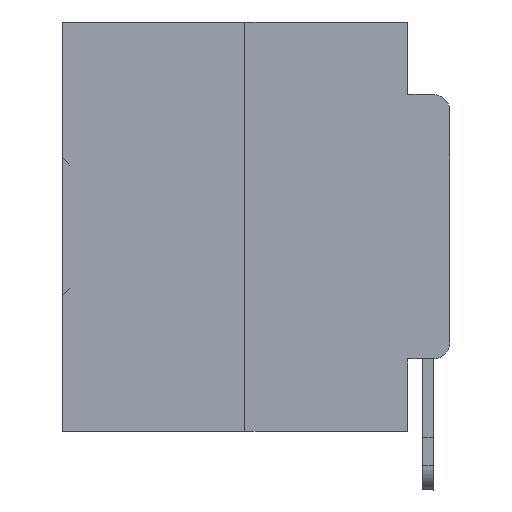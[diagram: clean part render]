
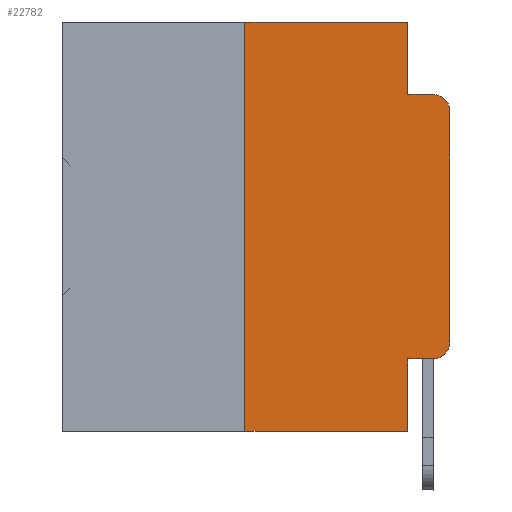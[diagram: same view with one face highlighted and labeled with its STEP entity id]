
A CAD part, left-side view. The second image highlights one B-rep face of the part: STEP entity #22782.
In plain terms, the highlighted planar face has unit normal (-1, 0, 0).
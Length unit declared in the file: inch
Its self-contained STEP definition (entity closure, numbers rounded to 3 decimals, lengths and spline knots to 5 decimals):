
#149 = CARTESIAN_POINT ( 'NONE',  ( 0., 0.051, -0.4115 ) ) ;
#343 = VERTEX_POINT ( 'NONE', #36033 ) ;
#1780 = CARTESIAN_POINT ( 'NONE',  ( 0., 0.051, 0. ) ) ;
#1832 = VECTOR ( 'NONE', #34281, 39.37008 ) ;
#2048 = EDGE_CURVE ( 'NONE', #2356, #4597, #19613, .T. ) ;
#2356 = VERTEX_POINT ( 'NONE', #21912 ) ;
#2500 = VERTEX_POINT ( 'NONE', #13783 ) ;
#2726 = ORIENTED_EDGE ( 'NONE', *, *, #29687, .F. ) ;
#3063 = ORIENTED_EDGE ( 'NONE', *, *, #31579, .F. ) ;
#3668 = EDGE_LOOP ( 'NONE', ( #34171, #30281, #2726, #24308, #3063, #38147, #25999, #22977, #11051, #19645 ) ) ;
#3927 = DIRECTION ( 'NONE',  ( 0., 0., -1. ) ) ;
#4092 = DIRECTION ( 'NONE',  ( -1., 0., 0. ) ) ;
#4597 = VERTEX_POINT ( 'NONE', #27988 ) ;
#5801 = VERTEX_POINT ( 'NONE', #20246 ) ;
#5892 = CARTESIAN_POINT ( 'NONE',  ( 0., 0.02, -0.0885 ) ) ;
#6077 = VECTOR ( 'NONE', #32406, 39.37008 ) ;
#6554 = DIRECTION ( 'NONE',  ( 1., 0., 0. ) ) ;
#7259 = AXIS2_PLACEMENT_3D ( 'NONE', #35576, #4092, #29789 ) ;
#7437 = CARTESIAN_POINT ( 'NONE',  ( 0., 0.051, -0.5 ) ) ;
#8068 = LINE ( 'NONE', #25431, #29196 ) ;
#8085 = EDGE_CURVE ( 'NONE', #11200, #343, #20637, .T. ) ;
#8087 = LINE ( 'NONE', #28728, #30565 ) ;
#8116 = VERTEX_POINT ( 'NONE', #9067 ) ;
#9067 = CARTESIAN_POINT ( 'NONE',  ( 0., 0.051, 0. ) ) ;
#9693 = LINE ( 'NONE', #36499, #15045 ) ;
#11051 = ORIENTED_EDGE ( 'NONE', *, *, #8085, .T. ) ;
#11105 = VECTOR ( 'NONE', #23665, 39.37008 ) ;
#11135 = CARTESIAN_POINT ( 'NONE',  ( 0., 0., 0. ) ) ;
#11200 = VERTEX_POINT ( 'NONE', #23392 ) ;
#12167 = AXIS2_PLACEMENT_3D ( 'NONE', #15905, #22455, #3927 ) ;
#12882 = CARTESIAN_POINT ( 'NONE',  ( 0., 0.051, -0.0885 ) ) ;
#13419 = CIRCLE ( 'NONE', #12167, 0.02 ) ;
#13783 = CARTESIAN_POINT ( 'NONE',  ( 0., 0.25, 0. ) ) ;
#13881 = VERTEX_POINT ( 'NONE', #5892 ) ;
#15045 = VECTOR ( 'NONE', #30336, 39.37008 ) ;
#15905 = CARTESIAN_POINT ( 'NONE',  ( 0., 0.02, -0.1085 ) ) ;
#17601 = VERTEX_POINT ( 'NONE', #12882 ) ;
#17665 = CARTESIAN_POINT ( 'NONE',  ( 0., 0.25, 0. ) ) ;
#18968 = DIRECTION ( 'NONE',  ( 0., 0., -1. ) ) ;
#19613 = LINE ( 'NONE', #11135, #1832 ) ;
#19645 = ORIENTED_EDGE ( 'NONE', *, *, #34532, .T. ) ;
#20246 = CARTESIAN_POINT ( 'NONE',  ( 0., 0.25, -0.5 ) ) ;
#20637 = LINE ( 'NONE', #149, #6077 ) ;
#20653 = DIRECTION ( 'NONE',  ( 0., 0., -1. ) ) ;
#21210 = VERTEX_POINT ( 'NONE', #7437 ) ;
#21238 = DIRECTION ( 'NONE',  ( 0., -1., 0. ) ) ;
#21912 = CARTESIAN_POINT ( 'NONE',  ( 0., 0., -0.3915 ) ) ;
#22017 = EDGE_CURVE ( 'NONE', #4597, #13881, #13419, .T. ) ;
#22455 = DIRECTION ( 'NONE',  ( -1., 0., 0. ) ) ;
#22782 = ADVANCED_FACE ( 'NONE', ( #30108 ), #24128, .F. ) ;
#22977 = ORIENTED_EDGE ( 'NONE', *, *, #28668, .F. ) ;
#23392 = CARTESIAN_POINT ( 'NONE',  ( 0., 0.051, -0.4115 ) ) ;
#23573 = LINE ( 'NONE', #32633, #33117 ) ;
#23665 = DIRECTION ( 'NONE',  ( 0., 0., 1. ) ) ;
#24128 = PLANE ( 'NONE',  #28870 ) ;
#24308 = ORIENTED_EDGE ( 'NONE', *, *, #26522, .F. ) ;
#24811 = VECTOR ( 'NONE', #18968, 39.37008 ) ;
#24882 = EDGE_CURVE ( 'NONE', #5801, #2500, #35063, .T. ) ;
#25431 = CARTESIAN_POINT ( 'NONE',  ( 0., 0.051, 0. ) ) ;
#25999 = ORIENTED_EDGE ( 'NONE', *, *, #32543, .T. ) ;
#26336 = DIRECTION ( 'NONE',  ( 0., 0., -1. ) ) ;
#26522 = EDGE_CURVE ( 'NONE', #8116, #17601, #36530, .T. ) ;
#27988 = CARTESIAN_POINT ( 'NONE',  ( 0., 0., -0.1085 ) ) ;
#28668 = EDGE_CURVE ( 'NONE', #11200, #21210, #8068, .T. ) ;
#28728 = CARTESIAN_POINT ( 'NONE',  ( 0., 0.473, 0. ) ) ;
#28870 = AXIS2_PLACEMENT_3D ( 'NONE', #35326, #6554, #20653 ) ;
#29196 = VECTOR ( 'NONE', #26336, 39.37008 ) ;
#29687 = EDGE_CURVE ( 'NONE', #17601, #13881, #9693, .T. ) ;
#29789 = DIRECTION ( 'NONE',  ( 0., 0., -1. ) ) ;
#30108 = FACE_OUTER_BOUND ( 'NONE', #3668, .T. ) ;
#30281 = ORIENTED_EDGE ( 'NONE', *, *, #22017, .T. ) ;
#30336 = DIRECTION ( 'NONE',  ( 0., -1., 0. ) ) ;
#30565 = VECTOR ( 'NONE', #37215, 39.37008 ) ;
#31579 = EDGE_CURVE ( 'NONE', #2500, #8116, #8087, .T. ) ;
#32406 = DIRECTION ( 'NONE',  ( 0., -1., 0. ) ) ;
#32543 = EDGE_CURVE ( 'NONE', #5801, #21210, #23573, .T. ) ;
#32633 = CARTESIAN_POINT ( 'NONE',  ( 0., 0.473, -0.5 ) ) ;
#33117 = VECTOR ( 'NONE', #21238, 39.37008 ) ;
#33141 = CIRCLE ( 'NONE', #7259, 0.02 ) ;
#34171 = ORIENTED_EDGE ( 'NONE', *, *, #2048, .T. ) ;
#34281 = DIRECTION ( 'NONE',  ( 0., 0., 1. ) ) ;
#34532 = EDGE_CURVE ( 'NONE', #343, #2356, #33141, .T. ) ;
#35063 = LINE ( 'NONE', #17665, #11105 ) ;
#35326 = CARTESIAN_POINT ( 'NONE',  ( 0., 0.473, 0. ) ) ;
#35576 = CARTESIAN_POINT ( 'NONE',  ( 0., 0.02, -0.3915 ) ) ;
#36033 = CARTESIAN_POINT ( 'NONE',  ( 0., 0.02, -0.4115 ) ) ;
#36499 = CARTESIAN_POINT ( 'NONE',  ( 0., 0.051, -0.0885 ) ) ;
#36530 = LINE ( 'NONE', #1780, #24811 ) ;
#37215 = DIRECTION ( 'NONE',  ( 0., -1., 0. ) ) ;
#38147 = ORIENTED_EDGE ( 'NONE', *, *, #24882, .F. ) ;
